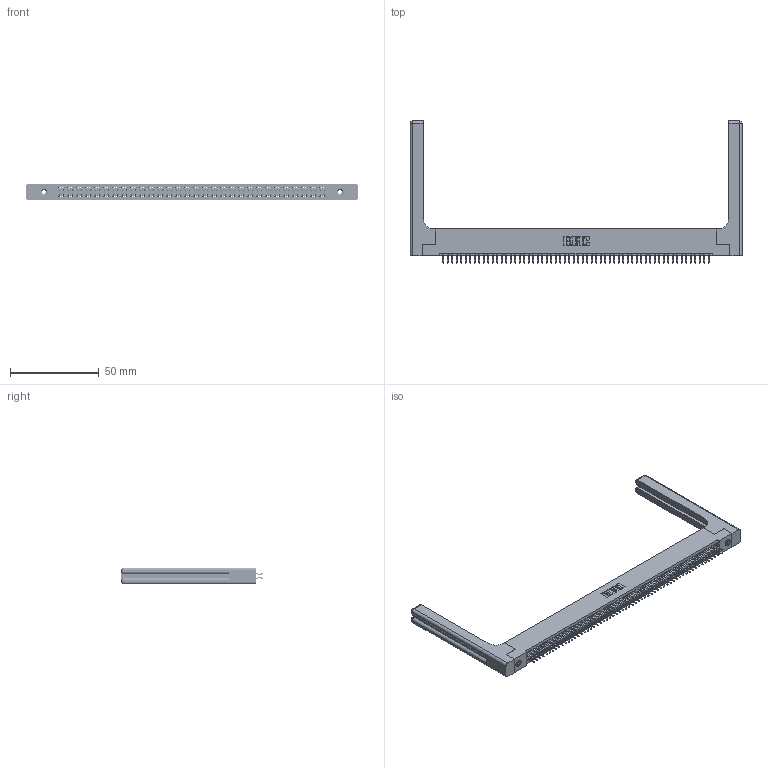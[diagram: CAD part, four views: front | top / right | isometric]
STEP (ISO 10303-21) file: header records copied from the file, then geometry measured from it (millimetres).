
FILE_DESCRIPTION (( 'STEP AP203' ), '1' );
FILE_NAME ('345-120-556-258.STEP', '2019-11-06T03:34:03', ( '' ), ( '' ), 'SwSTEP 2.0', 'SolidWorks 2016', '' );
FILE_SCHEMA (( 'CONFIG_CONTROL_DESIGN' ));
Length unit declared in the file: inch
Products named in the file (5): 345-250-001_345-250-001-102; 345-292-001_556 Tail; 345-120-556-258; 345-220-058_345-220-058; 345 Part_Flush Mounting Lugs - 0.156 Dia-TH
Assembly tree (125 placements, depth 2):
  345-120-556-258
    345 Part_Flush Mounting Lugs - 0.156 Dia-TH
    345-292-001_556 Tail  x120
    345-250-001_345-250-001-102  x2
    345-220-058_345-220-058  x2
Bounding box: 187.43 x 80.2 x 9.4 mm (x, y, z)
Volume: 26844.3 mm3; surface area: 32455.1 mm2
Topology: 125 solids, 125 shells, 7102 faces, 21047 edges, 13850 vertices
Faces by surface type: plane 4668, cylinder 2374, bspline 36, cone 12, sphere 8, torus 4
Entity records: 50056 total; most frequent: CARTESIAN_POINT 9381, ORIENTED_EDGE 8100, DIRECTION 7170, EDGE_CURVE 4050, LINE 3578, VECTOR 3578, VERTEX_POINT 2690, AXIS2_PLACEMENT_3D 1796
